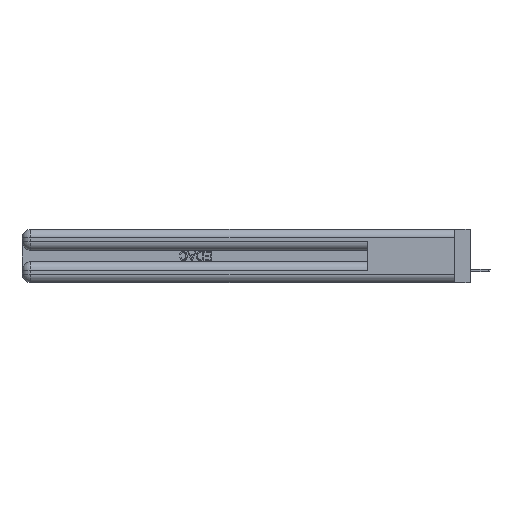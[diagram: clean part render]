
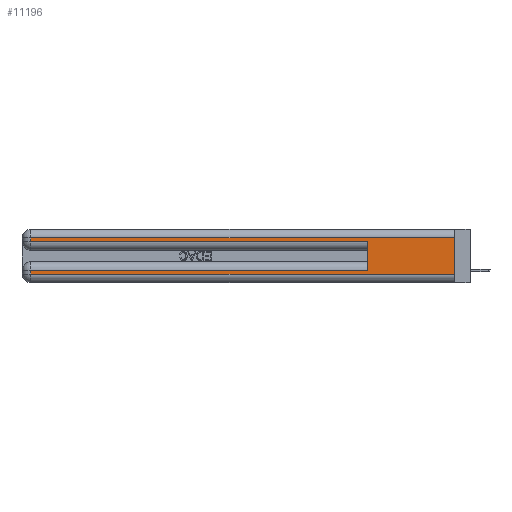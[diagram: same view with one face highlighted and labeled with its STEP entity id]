
A CAD part, left-side view. The second image highlights one B-rep face of the part: STEP entity #11196.
In plain terms, the highlighted planar face has unit normal (-1, 0, 0).
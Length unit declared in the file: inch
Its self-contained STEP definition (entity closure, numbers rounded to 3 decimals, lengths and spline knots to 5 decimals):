
#602 = LINE ( 'NONE', #35735, #2162 ) ;
#2162 = VECTOR ( 'NONE', #45276, 39.37008 ) ;
#2174 = LINE ( 'NONE', #53595, #4525 ) ;
#2369 = CARTESIAN_POINT ( 'NONE',  ( 0., 2.94, 0.085 ) ) ;
#2905 = CARTESIAN_POINT ( 'NONE',  ( 0., 0., 0.06 ) ) ;
#4525 = VECTOR ( 'NONE', #11916, 39.37008 ) ;
#4721 = ORIENTED_EDGE ( 'NONE', *, *, #7366, .T. ) ;
#5182 = LINE ( 'NONE', #47634, #18317 ) ;
#5379 = LINE ( 'NONE', #5939, #32120 ) ;
#5939 = CARTESIAN_POINT ( 'NONE',  ( 0., 0.6, 0.145 ) ) ;
#6413 = DIRECTION ( 'NONE',  ( 0., -1., 0. ) ) ;
#6531 = ORIENTED_EDGE ( 'NONE', *, *, #54632, .F. ) ;
#6741 = ORIENTED_EDGE ( 'NONE', *, *, #18823, .T. ) ;
#7366 = EDGE_CURVE ( 'NONE', #26345, #13706, #16551, .T. ) ;
#8037 = VECTOR ( 'NONE', #21013, 39.37008 ) ;
#8070 = LINE ( 'NONE', #11451, #8037 ) ;
#8811 = CARTESIAN_POINT ( 'NONE',  ( 0., 0., 0.37 ) ) ;
#9404 = DIRECTION ( 'NONE',  ( 0., 1., 0. ) ) ;
#9735 = VERTEX_POINT ( 'NONE', #23721 ) ;
#9771 = VECTOR ( 'NONE', #6413, 39.37008 ) ;
#10620 = LINE ( 'NONE', #53884, #9771 ) ;
#11196 = ADVANCED_FACE ( 'NONE', ( #13030 ), #47322, .F. ) ;
#11451 = CARTESIAN_POINT ( 'NONE',  ( 0., 2.94, 0.37 ) ) ;
#11636 = ORIENTED_EDGE ( 'NONE', *, *, #17030, .T. ) ;
#11873 = VERTEX_POINT ( 'NONE', #53653 ) ;
#11916 = DIRECTION ( 'NONE',  ( 0., 0., -1. ) ) ;
#13030 = FACE_OUTER_BOUND ( 'NONE', #36151, .T. ) ;
#13540 = ORIENTED_EDGE ( 'NONE', *, *, #22934, .F. ) ;
#13706 = VERTEX_POINT ( 'NONE', #32796 ) ;
#16551 = LINE ( 'NONE', #39320, #51408 ) ;
#17030 = EDGE_CURVE ( 'NONE', #50872, #35011, #602, .T. ) ;
#17284 = LINE ( 'NONE', #33325, #35624 ) ;
#18317 = VECTOR ( 'NONE', #9404, 39.37008 ) ;
#18823 = EDGE_CURVE ( 'NONE', #9735, #50872, #5182, .T. ) ;
#21013 = DIRECTION ( 'NONE',  ( 0., 0., -1. ) ) ;
#22446 = DIRECTION ( 'NONE',  ( 0., 1., 0. ) ) ;
#22934 = EDGE_CURVE ( 'NONE', #9735, #11873, #5379, .T. ) ;
#23074 = DIRECTION ( 'NONE',  ( 0., 0., 1. ) ) ;
#23721 = CARTESIAN_POINT ( 'NONE',  ( 0., 0.6, 0.085 ) ) ;
#24834 = DIRECTION ( 'NONE',  ( 0., 0., -1. ) ) ;
#26345 = VERTEX_POINT ( 'NONE', #26918 ) ;
#26918 = CARTESIAN_POINT ( 'NONE',  ( 0., 0., 0.31 ) ) ;
#28966 = CARTESIAN_POINT ( 'NONE',  ( 0., 2.94, 0.06 ) ) ;
#29377 = EDGE_CURVE ( 'NONE', #35011, #48127, #10620, .T. ) ;
#30182 = EDGE_CURVE ( 'NONE', #13706, #38302, #8070, .T. ) ;
#32120 = VECTOR ( 'NONE', #23074, 39.37008 ) ;
#32796 = CARTESIAN_POINT ( 'NONE',  ( 0., 2.94, 0.31 ) ) ;
#33325 = CARTESIAN_POINT ( 'NONE',  ( 0., 0., 0.285 ) ) ;
#33471 = ORIENTED_EDGE ( 'NONE', *, *, #41553, .T. ) ;
#35011 = VERTEX_POINT ( 'NONE', #28966 ) ;
#35031 = AXIS2_PLACEMENT_3D ( 'NONE', #8811, #46210, #24834 ) ;
#35624 = VECTOR ( 'NONE', #47097, 39.37008 ) ;
#35735 = CARTESIAN_POINT ( 'NONE',  ( 0., 2.94, 0.37 ) ) ;
#36151 = EDGE_LOOP ( 'NONE', ( #6531, #4721, #47503, #33471, #13540, #6741, #11636, #48784 ) ) ;
#37335 = CARTESIAN_POINT ( 'NONE',  ( 0., 2.94, 0.285 ) ) ;
#38302 = VERTEX_POINT ( 'NONE', #37335 ) ;
#39320 = CARTESIAN_POINT ( 'NONE',  ( 0., 0., 0.31 ) ) ;
#41553 = EDGE_CURVE ( 'NONE', #38302, #11873, #17284, .T. ) ;
#45276 = DIRECTION ( 'NONE',  ( 0., 0., -1. ) ) ;
#46210 = DIRECTION ( 'NONE',  ( 1., 0., 0. ) ) ;
#47097 = DIRECTION ( 'NONE',  ( 0., -1., 0. ) ) ;
#47322 = PLANE ( 'NONE',  #35031 ) ;
#47503 = ORIENTED_EDGE ( 'NONE', *, *, #30182, .T. ) ;
#47634 = CARTESIAN_POINT ( 'NONE',  ( 0., 0., 0.085 ) ) ;
#48127 = VERTEX_POINT ( 'NONE', #2905 ) ;
#48784 = ORIENTED_EDGE ( 'NONE', *, *, #29377, .T. ) ;
#50872 = VERTEX_POINT ( 'NONE', #2369 ) ;
#51408 = VECTOR ( 'NONE', #22446, 39.37008 ) ;
#53595 = CARTESIAN_POINT ( 'NONE',  ( 0., 0., 0.37 ) ) ;
#53653 = CARTESIAN_POINT ( 'NONE',  ( 0., 0.6, 0.285 ) ) ;
#53884 = CARTESIAN_POINT ( 'NONE',  ( 0., 0., 0.06 ) ) ;
#54632 = EDGE_CURVE ( 'NONE', #26345, #48127, #2174, .T. ) ;
